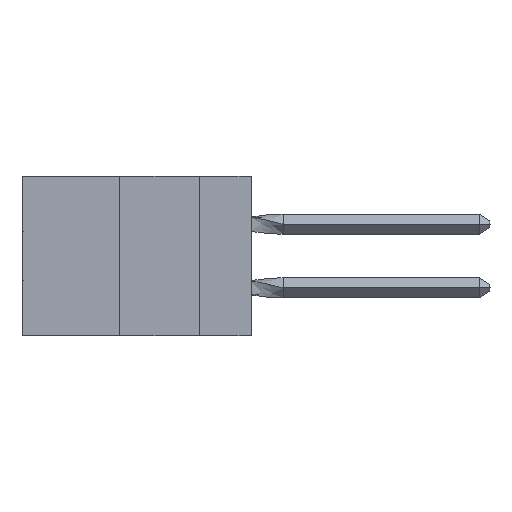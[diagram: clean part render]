
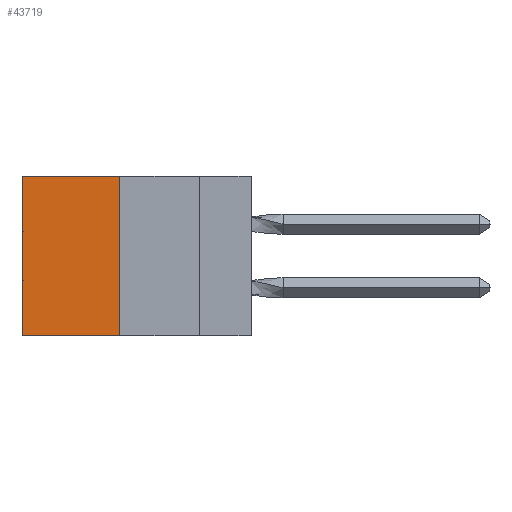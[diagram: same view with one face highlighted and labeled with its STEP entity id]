
A CAD part, left-side view. The second image highlights one B-rep face of the part: STEP entity #43719.
In plain terms, the highlighted planar face has unit normal (-1, 0, 0).
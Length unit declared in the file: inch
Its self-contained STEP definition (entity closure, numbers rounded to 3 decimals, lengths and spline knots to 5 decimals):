
#1676 = VECTOR ( 'NONE', #26462, 39.37008 ) ;
#1760 = EDGE_CURVE ( 'NONE', #30272, #32542, #9017, .T. ) ;
#3169 = LINE ( 'NONE', #20354, #20213 ) ;
#4791 = CARTESIAN_POINT ( 'NONE',  ( 0.305, 0.413, -0.5 ) ) ;
#5542 = DIRECTION ( 'NONE',  ( 0., 1., 0. ) ) ;
#6055 = ORIENTED_EDGE ( 'NONE', *, *, #37496, .T. ) ;
#7336 = VECTOR ( 'NONE', #5542, 39.37008 ) ;
#9017 = LINE ( 'NONE', #29030, #33941 ) ;
#11298 = EDGE_CURVE ( 'NONE', #32542, #41163, #31208, .T. ) ;
#12894 = LINE ( 'NONE', #26608, #1676 ) ;
#14136 = AXIS2_PLACEMENT_3D ( 'NONE', #16688, #37140, #36834 ) ;
#16688 = CARTESIAN_POINT ( 'NONE',  ( 0.305, 0.413, -0.5 ) ) ;
#18412 = EDGE_LOOP ( 'NONE', ( #6055, #18626, #19641, #28401 ) ) ;
#18626 = ORIENTED_EDGE ( 'NONE', *, *, #11298, .F. ) ;
#19641 = ORIENTED_EDGE ( 'NONE', *, *, #1760, .F. ) ;
#20213 = VECTOR ( 'NONE', #20640, 39.37008 ) ;
#20354 = CARTESIAN_POINT ( 'NONE',  ( 0.305, 0.413, 0. ) ) ;
#20640 = DIRECTION ( 'NONE',  ( 0., 1., 0. ) ) ;
#21559 = CARTESIAN_POINT ( 'NONE',  ( 0.305, 0.72, 0. ) ) ;
#21567 = VERTEX_POINT ( 'NONE', #21559 ) ;
#24958 = FACE_OUTER_BOUND ( 'NONE', #18412, .T. ) ;
#26462 = DIRECTION ( 'NONE',  ( 0., 0., -1. ) ) ;
#26608 = CARTESIAN_POINT ( 'NONE',  ( 0.305, 0.72, -0.5 ) ) ;
#28401 = ORIENTED_EDGE ( 'NONE', *, *, #43766, .T. ) ;
#28587 = DIRECTION ( 'NONE',  ( 0., 0., -1. ) ) ;
#29030 = CARTESIAN_POINT ( 'NONE',  ( 0.305, 0.413, -0.5 ) ) ;
#30272 = VERTEX_POINT ( 'NONE', #43870 ) ;
#31208 = LINE ( 'NONE', #4791, #7336 ) ;
#32542 = VERTEX_POINT ( 'NONE', #34289 ) ;
#33270 = PLANE ( 'NONE',  #14136 ) ;
#33941 = VECTOR ( 'NONE', #28587, 39.37008 ) ;
#34289 = CARTESIAN_POINT ( 'NONE',  ( 0.305, 0.413, -0.5 ) ) ;
#36834 = DIRECTION ( 'NONE',  ( 0., 0., -1. ) ) ;
#37140 = DIRECTION ( 'NONE',  ( 1., 0., 0. ) ) ;
#37496 = EDGE_CURVE ( 'NONE', #21567, #41163, #12894, .T. ) ;
#41163 = VERTEX_POINT ( 'NONE', #43264 ) ;
#43264 = CARTESIAN_POINT ( 'NONE',  ( 0.305, 0.72, -0.5 ) ) ;
#43719 = ADVANCED_FACE ( 'NONE', ( #24958 ), #33270, .F. ) ;
#43766 = EDGE_CURVE ( 'NONE', #30272, #21567, #3169, .T. ) ;
#43870 = CARTESIAN_POINT ( 'NONE',  ( 0.305, 0.413, 0. ) ) ;
